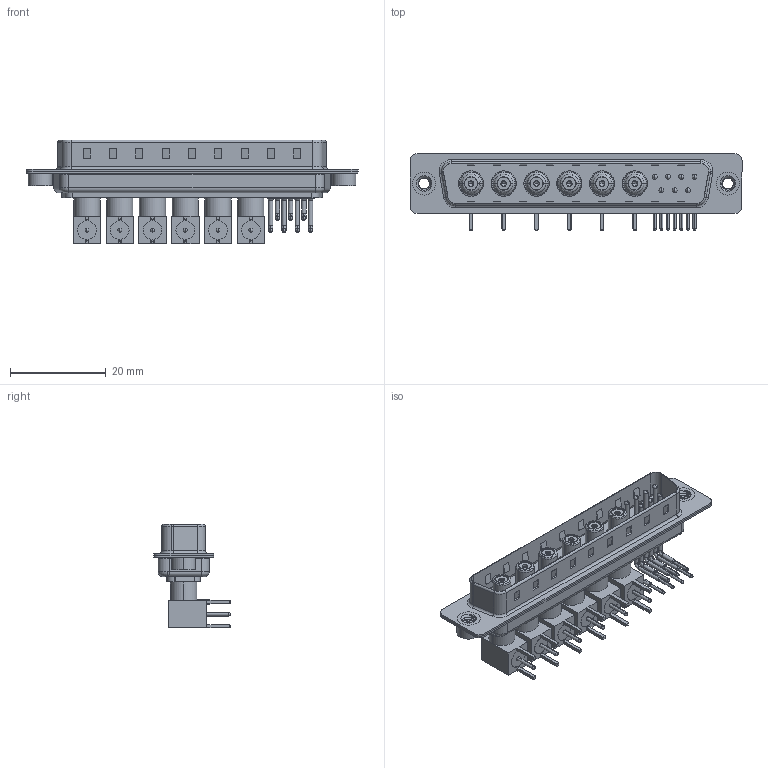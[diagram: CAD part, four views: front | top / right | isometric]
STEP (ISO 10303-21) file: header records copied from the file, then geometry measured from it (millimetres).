
FILE_DESCRIPTION (( 'STEP AP203' ), '1' );
FILE_NAME ('629-13W6640-5T2.STEP', '2022-05-14T18:50:42', ( '' ), ( '' ), 'SwSTEP 2.0', 'SolidWorks 2020', '' );
FILE_SCHEMA (( 'CONFIG_CONTROL_DESIGN' ));
Length unit declared in the file: millimetre
Products named in the file (20): Co-Ax Jack Assy_RA; 629Combo Shell Front_37 Contacts; Insulator Socket 2; 629Combo Shell Rear_37 Contacts; 629Combo Contact Row 1; Socket_RA; Locking Collar; Insulator RA Pin; Insulator Socket; 629Combo Threaded Rivet_2; 629Combo Contact Row 2; Co-Ax Jack_RA PC Tail; RA Back Shell; 629Combo Housing_13W6; 629-13W6640-5T2
Assembly tree (60 placements, depth 3):
  629-13W6640-5T2
    629Combo Housing_13W6
    629Combo Shell Rear_37 Contacts
    629Combo Shell Front_37 Contacts
    629Combo Threaded Rivet_2  x2
    Co-Ax Jack Assy_RA
      Co-Ax Jack_RA PC Tail
      Insulator Socket
      Insulator Socket 2
      Locking Collar
      Socket_RA
      RA Back Shell
      Insulator RA Pin
    Co-Ax Jack Assy_RA
      Co-Ax Jack_RA PC Tail
      Insulator Socket
      Insulator Socket 2
      Locking Collar
      Socket_RA
      RA Back Shell
      Insulator RA Pin
    Co-Ax Jack Assy_RA
      Co-Ax Jack_RA PC Tail
      Insulator Socket
      Insulator Socket 2
      Locking Collar
      Socket_RA
      RA Back Shell
      Insulator RA Pin
    Co-Ax Jack Assy_RA
      Co-Ax Jack_RA PC Tail
      Insulator Socket
      Insulator Socket 2
      Locking Collar
      Socket_RA
      RA Back Shell
      Insulator RA Pin
    Co-Ax Jack Assy_RA
      Co-Ax Jack_RA PC Tail
      Insulator Socket
      Insulator Socket 2
      Locking Collar
      Socket_RA
      RA Back Shell
      Insulator RA Pin
    Co-Ax Jack Assy_RA
      Co-Ax Jack_RA PC Tail
      Insulator Socket
      Insulator Socket 2
      Locking Collar
      Socket_RA
      RA Back Shell
      Insulator RA Pin
    629Combo Contact Row 1  x4
    629Combo Contact Row 2  x3
Bounding box: 69.4 x 16 x 21.71 mm (x, y, z)
Volume: 5538 mm3; surface area: 14951 mm2
Topology: 54 solids, 54 shells, 2094 faces, 5305 edges, 3366 vertices
Faces by surface type: plane 993, cylinder 795, cone 154, torus 86, bspline 54, sphere 12
Entity records: 29947 total; most frequent: CARTESIAN_POINT 6199, DIRECTION 4478, ORIENTED_EDGE 4146, EDGE_CURVE 2073, AXIS2_PLACEMENT_3D 1601, VERTEX_POINT 1331, LINE 1276, VECTOR 1276
